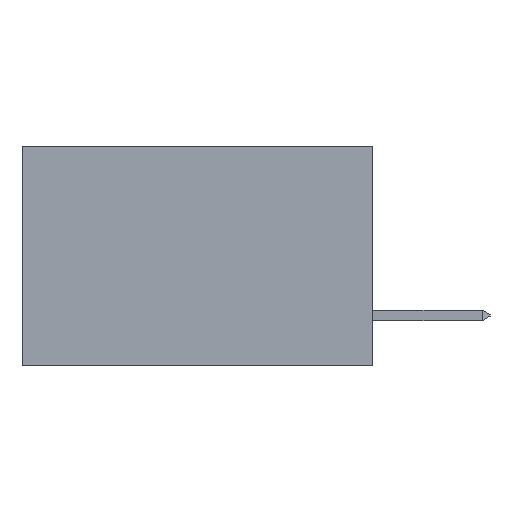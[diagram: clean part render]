
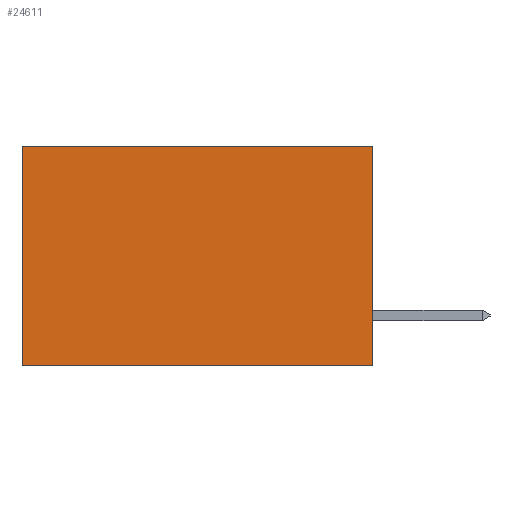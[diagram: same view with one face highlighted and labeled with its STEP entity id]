
A CAD part, left-side view. The second image highlights one B-rep face of the part: STEP entity #24611.
In plain terms, the highlighted planar face has unit normal (-1, 0, 0).
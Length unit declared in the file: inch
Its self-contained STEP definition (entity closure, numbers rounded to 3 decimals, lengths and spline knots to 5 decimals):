
#997 = DIRECTION ( 'NONE',  ( 0., 1., 0. ) ) ;
#2817 = CARTESIAN_POINT ( 'NONE',  ( 0.277, 0., -0.37 ) ) ;
#3250 = VECTOR ( 'NONE', #11500, 39.37008 ) ;
#3402 = PLANE ( 'NONE',  #23116 ) ;
#3704 = ORIENTED_EDGE ( 'NONE', *, *, #13657, .F. ) ;
#4050 = CARTESIAN_POINT ( 'NONE',  ( 0.277, 0.59, -0.37 ) ) ;
#4771 = EDGE_CURVE ( 'NONE', #7793, #11329, #8470, .T. ) ;
#5429 = DIRECTION ( 'NONE',  ( 1., 0., 0. ) ) ;
#5480 = VERTEX_POINT ( 'NONE', #15002 ) ;
#5508 = CARTESIAN_POINT ( 'NONE',  ( 0.277, 0., 0. ) ) ;
#6201 = LINE ( 'NONE', #2817, #15880 ) ;
#7793 = VERTEX_POINT ( 'NONE', #18954 ) ;
#8470 = LINE ( 'NONE', #5508, #3250 ) ;
#9752 = CARTESIAN_POINT ( 'NONE',  ( 0.277, 0.59, -0.37 ) ) ;
#11159 = EDGE_LOOP ( 'NONE', ( #23202, #18651, #3704, #14028 ) ) ;
#11329 = VERTEX_POINT ( 'NONE', #12609 ) ;
#11500 = DIRECTION ( 'NONE',  ( 0., 1., 0. ) ) ;
#11594 = LINE ( 'NONE', #4050, #16159 ) ;
#12609 = CARTESIAN_POINT ( 'NONE',  ( 0.277, 0.59, 0. ) ) ;
#12871 = CARTESIAN_POINT ( 'NONE',  ( 0.277, 0., -0.37 ) ) ;
#13657 = EDGE_CURVE ( 'NONE', #7793, #5480, #6201, .T. ) ;
#13693 = DIRECTION ( 'NONE',  ( 0., 0., -1. ) ) ;
#14028 = ORIENTED_EDGE ( 'NONE', *, *, #4771, .T. ) ;
#15002 = CARTESIAN_POINT ( 'NONE',  ( 0.277, 0., -0.37 ) ) ;
#15034 = CARTESIAN_POINT ( 'NONE',  ( 0.277, 0., -0.37 ) ) ;
#15350 = VECTOR ( 'NONE', #997, 39.37008 ) ;
#15880 = VECTOR ( 'NONE', #16563, 39.37008 ) ;
#16159 = VECTOR ( 'NONE', #13693, 39.37008 ) ;
#16563 = DIRECTION ( 'NONE',  ( 0., 0., -1. ) ) ;
#16607 = LINE ( 'NONE', #12871, #15350 ) ;
#16892 = EDGE_CURVE ( 'NONE', #5480, #18005, #16607, .T. ) ;
#18005 = VERTEX_POINT ( 'NONE', #9752 ) ;
#18651 = ORIENTED_EDGE ( 'NONE', *, *, #16892, .F. ) ;
#18954 = CARTESIAN_POINT ( 'NONE',  ( 0.277, 0., 0. ) ) ;
#18987 = DIRECTION ( 'NONE',  ( 0., 0., -1. ) ) ;
#23116 = AXIS2_PLACEMENT_3D ( 'NONE', #15034, #5429, #18987 ) ;
#23202 = ORIENTED_EDGE ( 'NONE', *, *, #24144, .T. ) ;
#24086 = FACE_OUTER_BOUND ( 'NONE', #11159, .T. ) ;
#24144 = EDGE_CURVE ( 'NONE', #11329, #18005, #11594, .T. ) ;
#24611 = ADVANCED_FACE ( 'NONE', ( #24086 ), #3402, .F. ) ;
